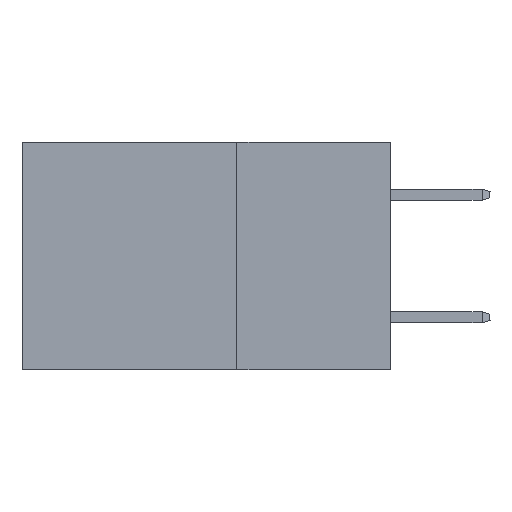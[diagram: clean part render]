
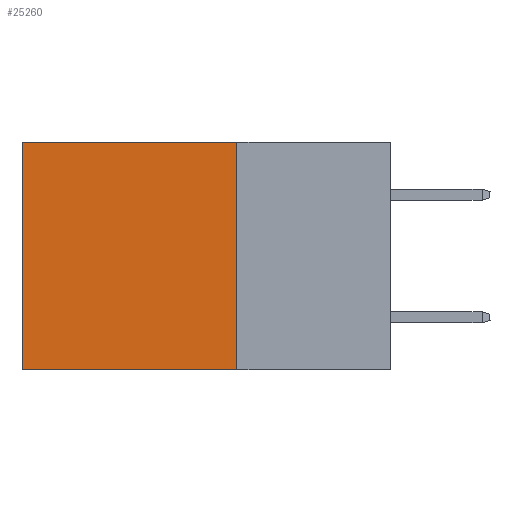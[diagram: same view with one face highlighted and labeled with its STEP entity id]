
A CAD part, left-side view. The second image highlights one B-rep face of the part: STEP entity #25260.
In plain terms, the highlighted planar face has unit normal (-1, 0, 0).
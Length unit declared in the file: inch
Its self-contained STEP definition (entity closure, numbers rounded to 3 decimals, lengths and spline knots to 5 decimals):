
#701 = FACE_OUTER_BOUND ( 'NONE', #26447, .T. ) ;
#837 = VERTEX_POINT ( 'NONE', #6865 ) ;
#883 = LINE ( 'NONE', #16514, #22677 ) ;
#916 = VERTEX_POINT ( 'NONE', #25580 ) ;
#1845 = CARTESIAN_POINT ( 'NONE',  ( 0.2875, 0.6, -0.37 ) ) ;
#3985 = VECTOR ( 'NONE', #38791, 39.37008 ) ;
#4374 = EDGE_CURVE ( 'NONE', #916, #38102, #24322, .T. ) ;
#6865 = CARTESIAN_POINT ( 'NONE',  ( 0.2875, 0.25, 0. ) ) ;
#7702 = EDGE_CURVE ( 'NONE', #837, #12007, #883, .T. ) ;
#10624 = DIRECTION ( 'NONE',  ( 0., 0., -1. ) ) ;
#11428 = EDGE_CURVE ( 'NONE', #837, #916, #32654, .T. ) ;
#12007 = VERTEX_POINT ( 'NONE', #13073 ) ;
#12672 = ORIENTED_EDGE ( 'NONE', *, *, #4374, .T. ) ;
#13073 = CARTESIAN_POINT ( 'NONE',  ( 0.2875, 0.25, -0.37 ) ) ;
#15752 = ORIENTED_EDGE ( 'NONE', *, *, #11428, .T. ) ;
#15932 = ORIENTED_EDGE ( 'NONE', *, *, #32855, .F. ) ;
#16514 = CARTESIAN_POINT ( 'NONE',  ( 0.2875, 0.25, 0. ) ) ;
#17596 = VECTOR ( 'NONE', #26024, 39.37008 ) ;
#20126 = CARTESIAN_POINT ( 'NONE',  ( 0.2875, 0.6, 0. ) ) ;
#22015 = VECTOR ( 'NONE', #38894, 39.37008 ) ;
#22677 = VECTOR ( 'NONE', #35202, 39.37008 ) ;
#22933 = PLANE ( 'NONE',  #28365 ) ;
#24322 = LINE ( 'NONE', #20126, #3985 ) ;
#25260 = ADVANCED_FACE ( 'NONE', ( #701 ), #22933, .F. ) ;
#25580 = CARTESIAN_POINT ( 'NONE',  ( 0.2875, 0.6, 0. ) ) ;
#26024 = DIRECTION ( 'NONE',  ( 0., 1., 0. ) ) ;
#26101 = DIRECTION ( 'NONE',  ( 1., 0., 0. ) ) ;
#26447 = EDGE_LOOP ( 'NONE', ( #12672, #15932, #30874, #15752 ) ) ;
#26509 = CARTESIAN_POINT ( 'NONE',  ( 0.2875, 0.25, -0.37 ) ) ;
#28365 = AXIS2_PLACEMENT_3D ( 'NONE', #29582, #26101, #10624 ) ;
#29582 = CARTESIAN_POINT ( 'NONE',  ( 0.2875, 0.25, 0. ) ) ;
#30874 = ORIENTED_EDGE ( 'NONE', *, *, #7702, .F. ) ;
#32654 = LINE ( 'NONE', #35560, #17596 ) ;
#32855 = EDGE_CURVE ( 'NONE', #12007, #38102, #34620, .T. ) ;
#34620 = LINE ( 'NONE', #26509, #22015 ) ;
#35202 = DIRECTION ( 'NONE',  ( 0., 0., -1. ) ) ;
#35560 = CARTESIAN_POINT ( 'NONE',  ( 0.2875, 0.25, 0. ) ) ;
#38102 = VERTEX_POINT ( 'NONE', #1845 ) ;
#38791 = DIRECTION ( 'NONE',  ( 0., 0., -1. ) ) ;
#38894 = DIRECTION ( 'NONE',  ( 0., 1., 0. ) ) ;
